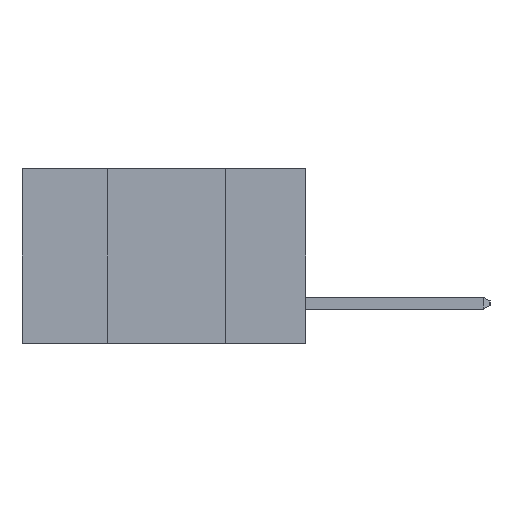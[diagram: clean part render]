
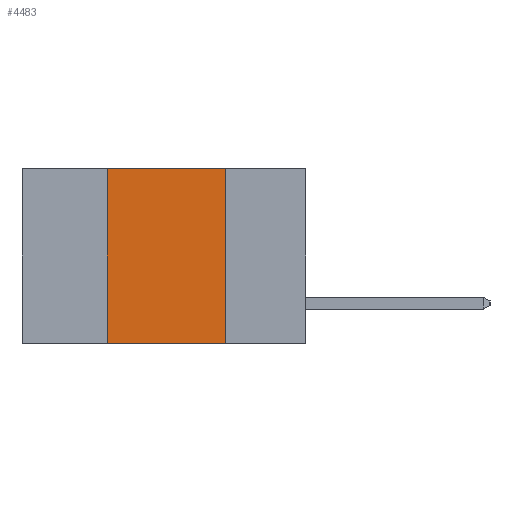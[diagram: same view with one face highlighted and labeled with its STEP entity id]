
A CAD part, left-side view. The second image highlights one B-rep face of the part: STEP entity #4483.
In plain terms, the highlighted planar face has unit normal (-1, 0, 0).
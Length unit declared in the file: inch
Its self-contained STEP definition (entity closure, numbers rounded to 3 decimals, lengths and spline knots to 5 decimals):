
#75 = EDGE_LOOP ( 'NONE', ( #5383, #4887, #2631, #5776 ) ) ;
#309 = CARTESIAN_POINT ( 'NONE',  ( 0., 0.42, -0.37 ) ) ;
#316 = DIRECTION ( 'NONE',  ( 0., 0., -1. ) ) ;
#784 = CARTESIAN_POINT ( 'NONE',  ( 0., 0.42, -0.37 ) ) ;
#970 = VECTOR ( 'NONE', #1287, 39.37008 ) ;
#1287 = DIRECTION ( 'NONE',  ( 0., -1., 0. ) ) ;
#1439 = CARTESIAN_POINT ( 'NONE',  ( 0., 0.17, -0.37 ) ) ;
#1662 = CARTESIAN_POINT ( 'NONE',  ( 0., 0.17, -0.37 ) ) ;
#2162 = VERTEX_POINT ( 'NONE', #8072 ) ;
#2275 = DIRECTION ( 'NONE',  ( 0., 0., 1. ) ) ;
#2298 = CARTESIAN_POINT ( 'NONE',  ( 0., 0.6, -0.37 ) ) ;
#2404 = EDGE_CURVE ( 'NONE', #2162, #4685, #5183, .T. ) ;
#2631 = ORIENTED_EDGE ( 'NONE', *, *, #4729, .F. ) ;
#3767 = VERTEX_POINT ( 'NONE', #6721 ) ;
#4124 = LINE ( 'NONE', #2298, #7708 ) ;
#4483 = ADVANCED_FACE ( 'NONE', ( #8486 ), #4792, .F. ) ;
#4494 = EDGE_CURVE ( 'NONE', #3767, #2162, #6749, .T. ) ;
#4685 = VERTEX_POINT ( 'NONE', #1439 ) ;
#4729 = EDGE_CURVE ( 'NONE', #5507, #3767, #8790, .T. ) ;
#4792 = PLANE ( 'NONE',  #9181 ) ;
#4887 = ORIENTED_EDGE ( 'NONE', *, *, #4494, .F. ) ;
#4955 = VECTOR ( 'NONE', #316, 39.37008 ) ;
#5183 = LINE ( 'NONE', #1662, #4955 ) ;
#5383 = ORIENTED_EDGE ( 'NONE', *, *, #2404, .F. ) ;
#5507 = VERTEX_POINT ( 'NONE', #309 ) ;
#5776 = ORIENTED_EDGE ( 'NONE', *, *, #8453, .T. ) ;
#6442 = DIRECTION ( 'NONE',  ( 1., 0., 0. ) ) ;
#6451 = CARTESIAN_POINT ( 'NONE',  ( 0., 0.6, 0. ) ) ;
#6577 = DIRECTION ( 'NONE',  ( 0., 0., -1. ) ) ;
#6721 = CARTESIAN_POINT ( 'NONE',  ( 0., 0.42, 0. ) ) ;
#6749 = LINE ( 'NONE', #7453, #970 ) ;
#6842 = DIRECTION ( 'NONE',  ( 0., -1., 0. ) ) ;
#7453 = CARTESIAN_POINT ( 'NONE',  ( 0., 0.6, 0. ) ) ;
#7708 = VECTOR ( 'NONE', #6842, 39.37008 ) ;
#8072 = CARTESIAN_POINT ( 'NONE',  ( 0., 0.17, 0. ) ) ;
#8453 = EDGE_CURVE ( 'NONE', #5507, #4685, #4124, .T. ) ;
#8486 = FACE_OUTER_BOUND ( 'NONE', #75, .T. ) ;
#8586 = VECTOR ( 'NONE', #2275, 39.37008 ) ;
#8790 = LINE ( 'NONE', #784, #8586 ) ;
#9181 = AXIS2_PLACEMENT_3D ( 'NONE', #6451, #6442, #6577 ) ;
